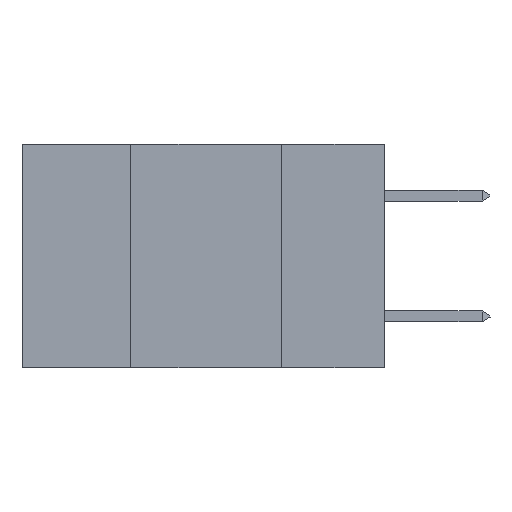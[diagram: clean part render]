
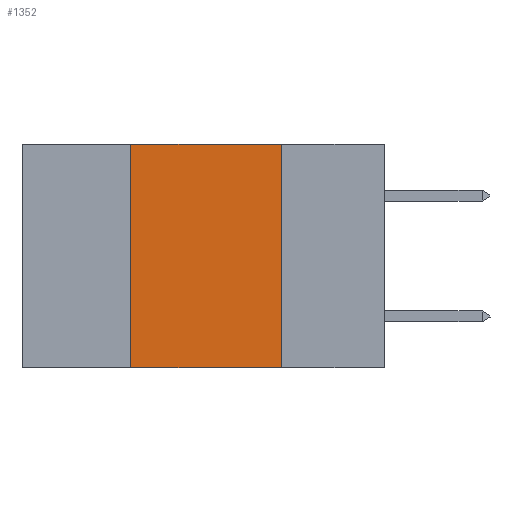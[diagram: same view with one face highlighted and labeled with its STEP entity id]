
A CAD part, left-side view. The second image highlights one B-rep face of the part: STEP entity #1352.
In plain terms, the highlighted planar face has unit normal (-1, 0, 0).
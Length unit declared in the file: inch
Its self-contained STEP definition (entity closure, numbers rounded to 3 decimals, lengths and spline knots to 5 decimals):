
#177 = VERTEX_POINT ( 'NONE', #11936 ) ;
#375 = ORIENTED_EDGE ( 'NONE', *, *, #15024, .F. ) ;
#800 = DIRECTION ( 'NONE',  ( 0., -1., 0. ) ) ;
#1115 = DIRECTION ( 'NONE',  ( 0., 0., 1. ) ) ;
#1352 = ADVANCED_FACE ( 'NONE', ( #12150 ), #2983, .F. ) ;
#1588 = DIRECTION ( 'NONE',  ( 1., 0., 0. ) ) ;
#1772 = LINE ( 'NONE', #6716, #2007 ) ;
#2007 = VECTOR ( 'NONE', #9692, 39.37008 ) ;
#2725 = VERTEX_POINT ( 'NONE', #15918 ) ;
#2983 = PLANE ( 'NONE',  #12401 ) ;
#4671 = ORIENTED_EDGE ( 'NONE', *, *, #12972, .F. ) ;
#5027 = LINE ( 'NONE', #7045, #8374 ) ;
#5667 = LINE ( 'NONE', #6603, #12976 ) ;
#6146 = VECTOR ( 'NONE', #8510, 39.37008 ) ;
#6451 = DIRECTION ( 'NONE',  ( 0., 0., -1. ) ) ;
#6603 = CARTESIAN_POINT ( 'NONE',  ( 0., 0.6, 0. ) ) ;
#6716 = CARTESIAN_POINT ( 'NONE',  ( 0., 0.17, 0. ) ) ;
#7045 = CARTESIAN_POINT ( 'NONE',  ( 0., 0.42, 0. ) ) ;
#8374 = VECTOR ( 'NONE', #1115, 39.37008 ) ;
#8510 = DIRECTION ( 'NONE',  ( 0., -1., 0. ) ) ;
#8611 = CARTESIAN_POINT ( 'NONE',  ( 0., 0.42, -0.37 ) ) ;
#9692 = DIRECTION ( 'NONE',  ( 0., 0., -1. ) ) ;
#10223 = VERTEX_POINT ( 'NONE', #8611 ) ;
#10400 = EDGE_CURVE ( 'NONE', #10223, #12931, #18593, .T. ) ;
#11936 = CARTESIAN_POINT ( 'NONE',  ( 0., 0.17, 0. ) ) ;
#12150 = FACE_OUTER_BOUND ( 'NONE', #16618, .T. ) ;
#12401 = AXIS2_PLACEMENT_3D ( 'NONE', #16680, #1588, #6451 ) ;
#12931 = VERTEX_POINT ( 'NONE', #19000 ) ;
#12972 = EDGE_CURVE ( 'NONE', #177, #12931, #1772, .T. ) ;
#12976 = VECTOR ( 'NONE', #800, 39.37008 ) ;
#14268 = ORIENTED_EDGE ( 'NONE', *, *, #10400, .T. ) ;
#15024 = EDGE_CURVE ( 'NONE', #10223, #2725, #5027, .T. ) ;
#15918 = CARTESIAN_POINT ( 'NONE',  ( 0., 0.42, 0. ) ) ;
#15935 = CARTESIAN_POINT ( 'NONE',  ( 0., 0.6, -0.37 ) ) ;
#16618 = EDGE_LOOP ( 'NONE', ( #4671, #17620, #375, #14268 ) ) ;
#16680 = CARTESIAN_POINT ( 'NONE',  ( 0., 0.6, 0. ) ) ;
#17620 = ORIENTED_EDGE ( 'NONE', *, *, #18360, .F. ) ;
#18360 = EDGE_CURVE ( 'NONE', #2725, #177, #5667, .T. ) ;
#18593 = LINE ( 'NONE', #15935, #6146 ) ;
#19000 = CARTESIAN_POINT ( 'NONE',  ( 0., 0.17, -0.37 ) ) ;
